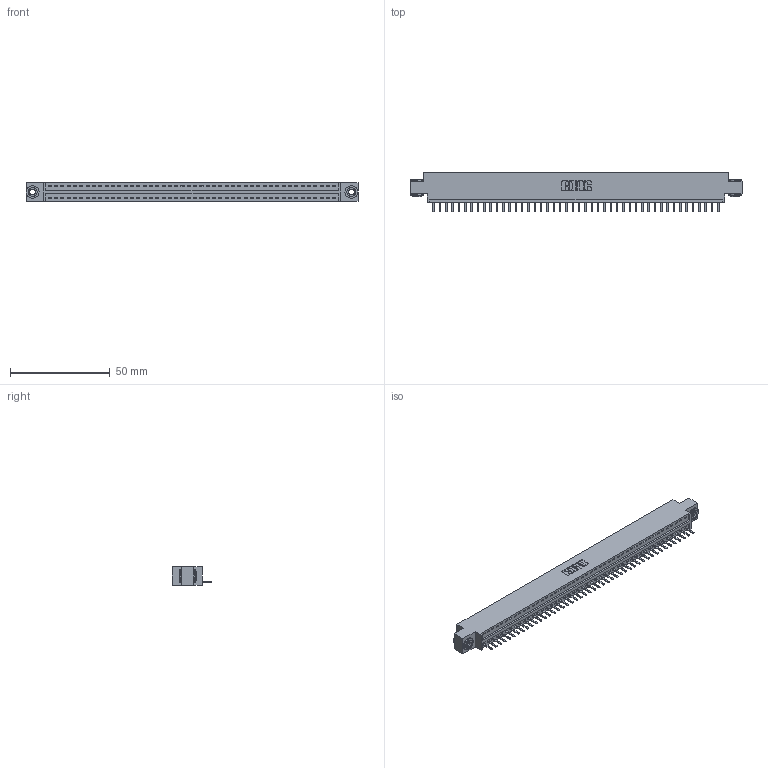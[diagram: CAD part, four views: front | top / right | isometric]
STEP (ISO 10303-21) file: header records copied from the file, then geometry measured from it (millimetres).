
FILE_DESCRIPTION (( 'STEP AP203' ), '1' );
FILE_NAME ('396-046-520-603.STEP', '2018-09-07T07:13:57', ( '' ), ( '' ), 'SwSTEP 2.0', 'SolidWorks 2016', '' );
FILE_SCHEMA (( 'CONFIG_CONTROL_DESIGN' ));
Length unit declared in the file: inch
Products named in the file (4): 345-250-002_345-250-002-102; 396-046-520-603; 346 Part_0.170 Offset - 0.156 Dia-TH; 345-292-001_345-293-120
Assembly tree (49 placements, depth 2):
  396-046-520-603
    346 Part_0.170 Offset - 0.156 Dia-TH
    345-292-001_345-293-120  x46
    345-250-002_345-250-002-102  x2
Bounding box: 166.62 x 20.02 x 9.4 mm (x, y, z)
Volume: 15709.6 mm3; surface area: 19616 mm2
Topology: 49 solids, 49 shells, 3016 faces, 8881 edges, 5794 vertices
Faces by surface type: plane 2022, cylinder 986, cone 8
Entity records: 28906 total; most frequent: CARTESIAN_POINT 4945, ORIENTED_EDGE 4906, DIRECTION 4375, EDGE_CURVE 2453, VECTOR 2109, LINE 2109, VERTEX_POINT 1630, AXIS2_PLACEMENT_3D 1133
